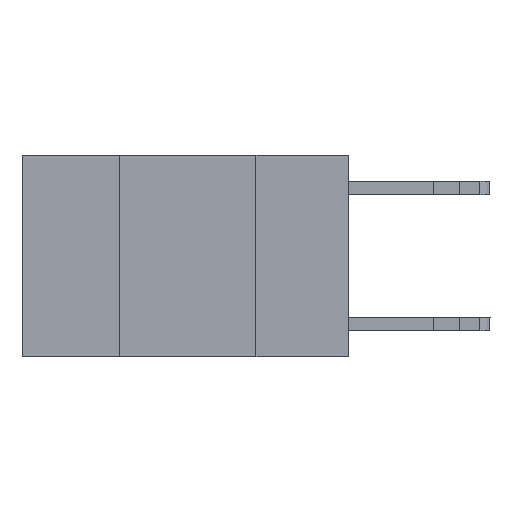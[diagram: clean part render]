
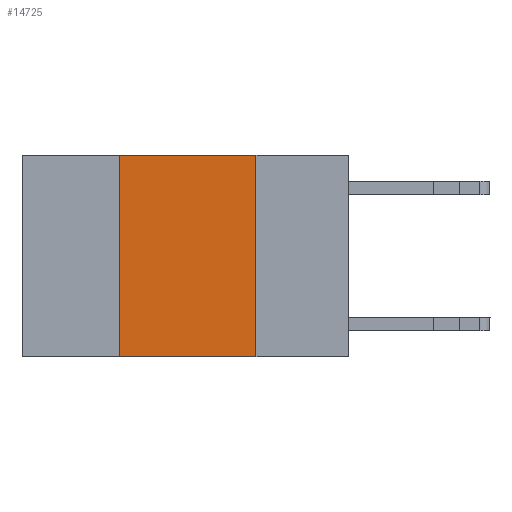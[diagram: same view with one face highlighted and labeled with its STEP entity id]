
A CAD part, left-side view. The second image highlights one B-rep face of the part: STEP entity #14725.
In plain terms, the highlighted planar face has unit normal (-1, 0, 0).
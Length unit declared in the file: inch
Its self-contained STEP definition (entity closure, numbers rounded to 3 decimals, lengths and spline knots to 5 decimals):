
#105 = CARTESIAN_POINT ( 'NONE',  ( 0., 0.42, 0. ) ) ;
#250 = DIRECTION ( 'NONE',  ( 0., 0., 1. ) ) ;
#310 = CARTESIAN_POINT ( 'NONE',  ( 0., 0.42, 0. ) ) ;
#653 = FACE_OUTER_BOUND ( 'NONE', #5575, .T. ) ;
#1981 = DIRECTION ( 'NONE',  ( 0., 0., -1. ) ) ;
#2104 = DIRECTION ( 'NONE',  ( 1., 0., 0. ) ) ;
#2290 = CARTESIAN_POINT ( 'NONE',  ( 0., 0.6, 0. ) ) ;
#2548 = PLANE ( 'NONE',  #11756 ) ;
#5575 = EDGE_LOOP ( 'NONE', ( #10793, #10508, #10592, #9840 ) ) ;
#8782 = EDGE_CURVE ( 'NONE', #18472, #12672, #19942, .T. ) ;
#8870 = VERTEX_POINT ( 'NONE', #18417 ) ;
#9840 = ORIENTED_EDGE ( 'NONE', *, *, #8782, .T. ) ;
#10508 = ORIENTED_EDGE ( 'NONE', *, *, #11461, .F. ) ;
#10592 = ORIENTED_EDGE ( 'NONE', *, *, #11073, .F. ) ;
#10793 = ORIENTED_EDGE ( 'NONE', *, *, #12150, .F. ) ;
#11073 = EDGE_CURVE ( 'NONE', #18472, #12022, #20879, .T. ) ;
#11461 = EDGE_CURVE ( 'NONE', #12022, #8870, #19061, .T. ) ;
#11756 = AXIS2_PLACEMENT_3D ( 'NONE', #2290, #2104, #1981 ) ;
#12022 = VERTEX_POINT ( 'NONE', #105 ) ;
#12150 = EDGE_CURVE ( 'NONE', #8870, #12672, #15292, .T. ) ;
#12672 = VERTEX_POINT ( 'NONE', #20615 ) ;
#14725 = ADVANCED_FACE ( 'NONE', ( #653 ), #2548, .F. ) ;
#15201 = VECTOR ( 'NONE', #17997, 39.37008 ) ;
#15292 = LINE ( 'NONE', #18367, #15201 ) ;
#17997 = DIRECTION ( 'NONE',  ( 0., 0., -1. ) ) ;
#18367 = CARTESIAN_POINT ( 'NONE',  ( 0., 0.17, 0. ) ) ;
#18417 = CARTESIAN_POINT ( 'NONE',  ( 0., 0.17, 0. ) ) ;
#18472 = VERTEX_POINT ( 'NONE', #20846 ) ;
#19002 = DIRECTION ( 'NONE',  ( 0., -1., 0. ) ) ;
#19044 = CARTESIAN_POINT ( 'NONE',  ( 0., 0.6, 0. ) ) ;
#19061 = LINE ( 'NONE', #19044, #19101 ) ;
#19101 = VECTOR ( 'NONE', #19002, 39.37008 ) ;
#19882 = VECTOR ( 'NONE', #19924, 39.37008 ) ;
#19924 = DIRECTION ( 'NONE',  ( 0., -1., 0. ) ) ;
#19942 = LINE ( 'NONE', #20813, #19882 ) ;
#20615 = CARTESIAN_POINT ( 'NONE',  ( 0., 0.17, -0.37 ) ) ;
#20813 = CARTESIAN_POINT ( 'NONE',  ( 0., 0.6, -0.37 ) ) ;
#20838 = VECTOR ( 'NONE', #250, 39.37008 ) ;
#20846 = CARTESIAN_POINT ( 'NONE',  ( 0., 0.42, -0.37 ) ) ;
#20879 = LINE ( 'NONE', #310, #20838 ) ;
